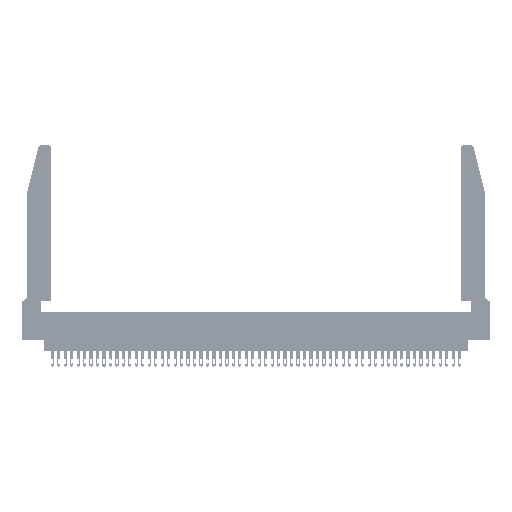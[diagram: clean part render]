
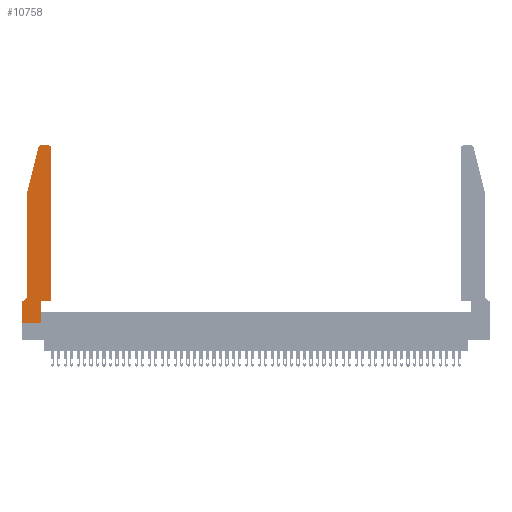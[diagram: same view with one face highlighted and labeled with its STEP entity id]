
A CAD part, top view. The second image highlights one B-rep face of the part: STEP entity #10758.
In plain terms, the highlighted planar face has unit normal (0, 0, 1).
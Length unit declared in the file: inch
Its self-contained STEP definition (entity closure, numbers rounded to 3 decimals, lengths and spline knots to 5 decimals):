
#249 = CARTESIAN_POINT ( 'NONE',  ( 0.0755, 0.42, 0.37 ) ) ;
#255 = AXIS2_PLACEMENT_3D ( 'NONE', #2884, #31015, #6566 ) ;
#2140 = EDGE_CURVE ( 'NONE', #19849, #40370, #28987, .T. ) ;
#2199 = DIRECTION ( 'NONE',  ( -0.239, -0.971, 0. ) ) ;
#2407 = PLANE ( 'NONE',  #20400 ) ;
#2884 = CARTESIAN_POINT ( 'NONE',  ( 0.0055, 0.42, 0.37 ) ) ;
#3389 = CARTESIAN_POINT ( 'NONE',  ( 0.284, 2.72, 0.37 ) ) ;
#5690 = VECTOR ( 'NONE', #2199, 39.37008 ) ;
#6046 = EDGE_CURVE ( 'NONE', #29989, #30326, #14404, .T. ) ;
#6438 = CARTESIAN_POINT ( 'NONE',  ( 0., 0.35, 0.37 ) ) ;
#6566 = DIRECTION ( 'NONE',  ( -1., 0., 0. ) ) ;
#6945 = ORIENTED_EDGE ( 'NONE', *, *, #37045, .T. ) ;
#7786 = ORIENTED_EDGE ( 'NONE', *, *, #15037, .T. ) ;
#7999 = LINE ( 'NONE', #45785, #33855 ) ;
#8293 = EDGE_CURVE ( 'NONE', #38252, #41930, #35336, .T. ) ;
#9152 = ORIENTED_EDGE ( 'NONE', *, *, #2140, .T. ) ;
#9432 = CARTESIAN_POINT ( 'NONE',  ( 0.4505, 0.35, 0.37 ) ) ;
#10271 = DIRECTION ( 'NONE',  ( 0., 1., 0. ) ) ;
#10758 = ADVANCED_FACE ( 'NONE', ( #21220 ), #2407, .T. ) ;
#11194 = DIRECTION ( 'NONE',  ( 1., 0., 0. ) ) ;
#11323 = DIRECTION ( 'NONE',  ( 1., 0., 0. ) ) ;
#11594 = ORIENTED_EDGE ( 'NONE', *, *, #12004, .T. ) ;
#11767 = CARTESIAN_POINT ( 'NONE',  ( 0.4205, 2.72, 0.37 ) ) ;
#12004 = EDGE_CURVE ( 'NONE', #23064, #12165, #24667, .T. ) ;
#12165 = VERTEX_POINT ( 'NONE', #45983 ) ;
#12796 = DIRECTION ( 'NONE',  ( 1., 0., 0. ) ) ;
#13421 = VERTEX_POINT ( 'NONE', #17247 ) ;
#14404 = LINE ( 'NONE', #15845, #46469 ) ;
#14481 = ORIENTED_EDGE ( 'NONE', *, *, #22037, .T. ) ;
#14878 = VECTOR ( 'NONE', #33905, 39.37008 ) ;
#15037 = EDGE_CURVE ( 'NONE', #42610, #37175, #25696, .T. ) ;
#15845 = CARTESIAN_POINT ( 'NONE',  ( 0., 0., 0.37 ) ) ;
#15928 = VECTOR ( 'NONE', #21481, 39.37008 ) ;
#16186 = CIRCLE ( 'NONE', #51331, 0.03 ) ;
#17182 = ORIENTED_EDGE ( 'NONE', *, *, #34111, .T. ) ;
#17247 = CARTESIAN_POINT ( 'NONE',  ( 0., 0.35, 0.37 ) ) ;
#17654 = CARTESIAN_POINT ( 'NONE',  ( 0.0755, 2., 0.37 ) ) ;
#17956 = ORIENTED_EDGE ( 'NONE', *, *, #43127, .T. ) ;
#18479 = CARTESIAN_POINT ( 'NONE',  ( 0., 0., 0.37 ) ) ;
#19699 = ORIENTED_EDGE ( 'NONE', *, *, #8293, .T. ) ;
#19805 = VECTOR ( 'NONE', #20719, 39.37008 ) ;
#19849 = VERTEX_POINT ( 'NONE', #52050 ) ;
#20400 = AXIS2_PLACEMENT_3D ( 'NONE', #6438, #34588, #11194 ) ;
#20719 = DIRECTION ( 'NONE',  ( -1., 0., 0. ) ) ;
#21064 = LINE ( 'NONE', #31280, #19805 ) ;
#21220 = FACE_OUTER_BOUND ( 'NONE', #34321, .T. ) ;
#21481 = DIRECTION ( 'NONE',  ( 0., -1., 0. ) ) ;
#22037 = EDGE_CURVE ( 'NONE', #37175, #13421, #21064, .T. ) ;
#22875 = EDGE_CURVE ( 'NONE', #40370, #42610, #29747, .T. ) ;
#23064 = VERTEX_POINT ( 'NONE', #39565 ) ;
#23314 = DIRECTION ( 'NONE',  ( 0., 0., 1. ) ) ;
#24667 = LINE ( 'NONE', #35987, #37254 ) ;
#25696 = CIRCLE ( 'NONE', #255, 0.07 ) ;
#25780 = DIRECTION ( 'NONE',  ( -1., 0., 0. ) ) ;
#25846 = CARTESIAN_POINT ( 'NONE',  ( 0.284, 2.75, 0.37 ) ) ;
#25891 = LINE ( 'NONE', #49164, #47257 ) ;
#26199 = EDGE_CURVE ( 'NONE', #30326, #23064, #7999, .T. ) ;
#27378 = VECTOR ( 'NONE', #50631, 39.37008 ) ;
#28987 = LINE ( 'NONE', #49414, #5690 ) ;
#29747 = LINE ( 'NONE', #17654, #15928 ) ;
#29989 = VERTEX_POINT ( 'NONE', #51388 ) ;
#30326 = VERTEX_POINT ( 'NONE', #45540 ) ;
#31015 = DIRECTION ( 'NONE',  ( 0., 0., -1. ) ) ;
#31280 = CARTESIAN_POINT ( 'NONE',  ( 0.0755, 0.35, 0.37 ) ) ;
#31955 = VERTEX_POINT ( 'NONE', #25846 ) ;
#32302 = CARTESIAN_POINT ( 'NONE',  ( 0.4505, 2.72, 0.37 ) ) ;
#32334 = CARTESIAN_POINT ( 'NONE',  ( 0.4205, 2.75, 0.37 ) ) ;
#32384 = ORIENTED_EDGE ( 'NONE', *, *, #26199, .T. ) ;
#32396 = ORIENTED_EDGE ( 'NONE', *, *, #43961, .T. ) ;
#33855 = VECTOR ( 'NONE', #10271, 39.37008 ) ;
#33905 = DIRECTION ( 'NONE',  ( 0., 1., 0. ) ) ;
#34111 = EDGE_CURVE ( 'NONE', #13421, #29989, #44938, .T. ) ;
#34321 = EDGE_LOOP ( 'NONE', ( #6945, #17956, #9152, #40714, #7786, #14481, #17182, #43158, #32384, #11594, #32396, #19699 ) ) ;
#34588 = DIRECTION ( 'NONE',  ( 0., 0., 1. ) ) ;
#35336 = CIRCLE ( 'NONE', #46266, 0.03 ) ;
#35987 = CARTESIAN_POINT ( 'NONE',  ( 0.4505, 0.35, 0.37 ) ) ;
#37045 = EDGE_CURVE ( 'NONE', #41930, #31955, #25891, .T. ) ;
#37175 = VERTEX_POINT ( 'NONE', #37872 ) ;
#37254 = VECTOR ( 'NONE', #12796, 39.37008 ) ;
#37872 = CARTESIAN_POINT ( 'NONE',  ( 0.0055, 0.35, 0.37 ) ) ;
#38252 = VERTEX_POINT ( 'NONE', #32302 ) ;
#39565 = CARTESIAN_POINT ( 'NONE',  ( 0.2865, 0.35, 0.37 ) ) ;
#40370 = VERTEX_POINT ( 'NONE', #49646 ) ;
#40714 = ORIENTED_EDGE ( 'NONE', *, *, #22875, .T. ) ;
#41930 = VERTEX_POINT ( 'NONE', #32334 ) ;
#42610 = VERTEX_POINT ( 'NONE', #249 ) ;
#43127 = EDGE_CURVE ( 'NONE', #31955, #19849, #16186, .T. ) ;
#43158 = ORIENTED_EDGE ( 'NONE', *, *, #6046, .T. ) ;
#43772 = DIRECTION ( 'NONE',  ( 0., 0., 1. ) ) ;
#43961 = EDGE_CURVE ( 'NONE', #12165, #38252, #46951, .T. ) ;
#44289 = DIRECTION ( 'NONE',  ( 1., 0., 0. ) ) ;
#44938 = LINE ( 'NONE', #18479, #27378 ) ;
#45540 = CARTESIAN_POINT ( 'NONE',  ( 0.2865, 0., 0.37 ) ) ;
#45785 = CARTESIAN_POINT ( 'NONE',  ( 0.2865, 0.35, 0.37 ) ) ;
#45983 = CARTESIAN_POINT ( 'NONE',  ( 0.4505, 0.35, 0.37 ) ) ;
#46266 = AXIS2_PLACEMENT_3D ( 'NONE', #11767, #43772, #51858 ) ;
#46469 = VECTOR ( 'NONE', #44289, 39.37008 ) ;
#46951 = LINE ( 'NONE', #9432, #14878 ) ;
#47257 = VECTOR ( 'NONE', #25780, 39.37008 ) ;
#49164 = CARTESIAN_POINT ( 'NONE',  ( 0.2605, 2.75, 0.37 ) ) ;
#49414 = CARTESIAN_POINT ( 'NONE',  ( 0.0755, 2., 0.37 ) ) ;
#49646 = CARTESIAN_POINT ( 'NONE',  ( 0.0755, 2., 0.37 ) ) ;
#50631 = DIRECTION ( 'NONE',  ( 0., -1., 0. ) ) ;
#51331 = AXIS2_PLACEMENT_3D ( 'NONE', #3389, #23314, #11323 ) ;
#51388 = CARTESIAN_POINT ( 'NONE',  ( 0., 0., 0.37 ) ) ;
#51858 = DIRECTION ( 'NONE',  ( 1., 0., 0. ) ) ;
#52050 = CARTESIAN_POINT ( 'NONE',  ( 0.25487, 2.72718, 0.37 ) ) ;
